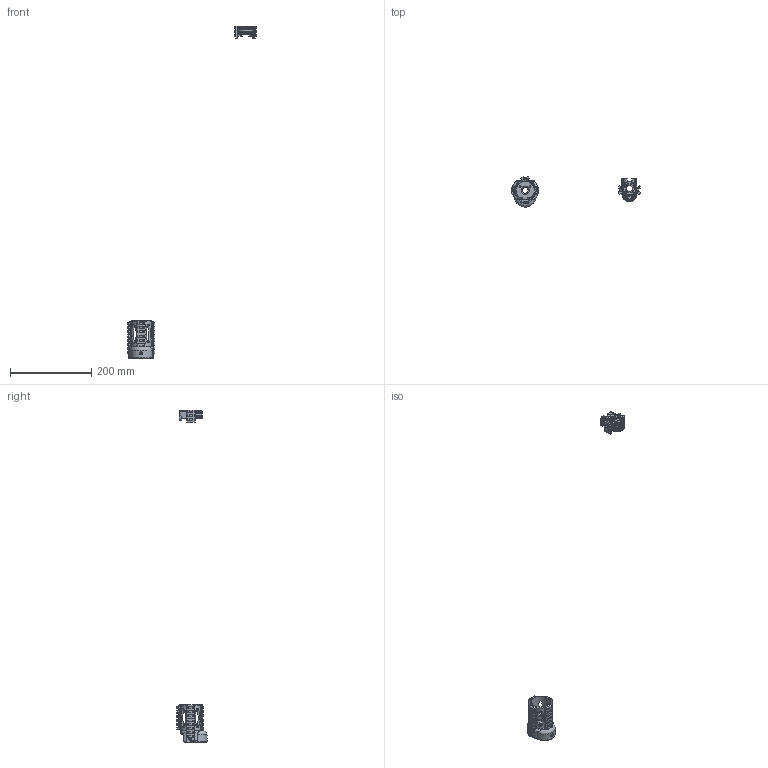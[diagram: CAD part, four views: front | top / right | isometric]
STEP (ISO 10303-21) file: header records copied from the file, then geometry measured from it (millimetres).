
FILE_DESCRIPTION(/* description */ (''),/* implementation_level */ '2;1');
FILE_NAME(/* name */ 'AP9 RAIL v7.step',/* time_stamp */ '2018-09-14T23:20:05-04:00',/* author */ (''),/* organization */ (''),/* preprocessor_version */ 'ST-DEVELOPER v17.2',/* originating_system */ 'Autodesk Translation Framework v7.6.0.251',/* authorisation */ '');
FILE_SCHEMA (('AUTOMOTIVE_DESIGN { 1 0 10303 214 3 1 1 }'));
Products named in the file (1): AP9 RAIL
Bounding box: 316.69 x 74 x 818.5 mm (x, y, z)
Volume: 154448.3 mm3; surface area: 51264 mm2
Topology: 2 solids, 3 shells, 4325 faces, 8198 edges, 3859 vertices
Faces by surface type: plane 4201, cylinder 60, bspline 47, torus 17
Full cylindrical faces by diameter (mm): 3.5 x4, 5 x3, 7 x2, 8 x2, 14.4 x1, 45 x1
Entity records: 103894 total; most frequent: CARTESIAN_POINT 19954, DIRECTION 17414, ORIENTED_EDGE 16454, EDGE_CURVE 8227, LINE 7288, VECTOR 7288, AXIS2_PLACEMENT_3D 5063, EDGE_LOOP 4343
